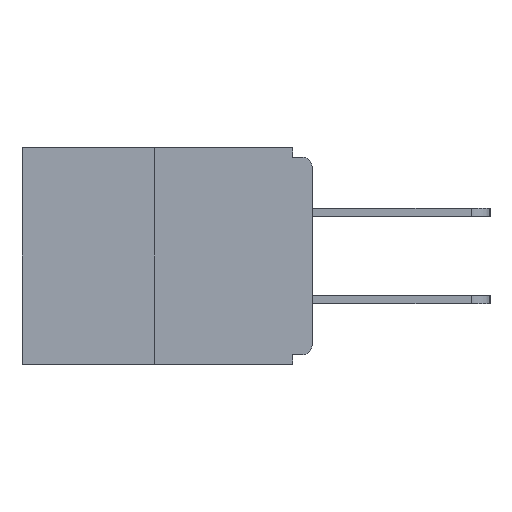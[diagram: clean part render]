
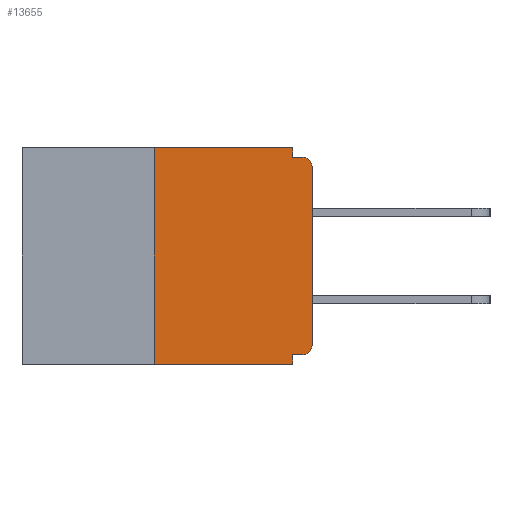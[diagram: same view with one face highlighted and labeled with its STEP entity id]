
A CAD part, left-side view. The second image highlights one B-rep face of the part: STEP entity #13655.
In plain terms, the highlighted planar face has unit normal (-1, 0, 0).
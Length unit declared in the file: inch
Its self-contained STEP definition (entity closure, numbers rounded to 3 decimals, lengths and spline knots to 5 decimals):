
#90 = VECTOR ( 'NONE', #7246, 39.37008 ) ;
#482 = CIRCLE ( 'NONE', #9554, 0.015 ) ;
#516 = DIRECTION ( 'NONE',  ( 0., 0., -1. ) ) ;
#605 = EDGE_CURVE ( 'NONE', #10616, #1938, #11566, .T. ) ;
#640 = PLANE ( 'NONE',  #7492 ) ;
#707 = EDGE_CURVE ( 'NONE', #5355, #6117, #7662, .T. ) ;
#779 = EDGE_CURVE ( 'NONE', #8005, #9842, #2909, .T. ) ;
#867 = ORIENTED_EDGE ( 'NONE', *, *, #605, .F. ) ;
#1139 = VECTOR ( 'NONE', #2866, 39.37008 ) ;
#1143 = ORIENTED_EDGE ( 'NONE', *, *, #3931, .F. ) ;
#1372 = CARTESIAN_POINT ( 'NONE',  ( 0., 0., -0.313 ) ) ;
#1499 = VECTOR ( 'NONE', #12798, 39.37008 ) ;
#1621 = CARTESIAN_POINT ( 'NONE',  ( 0., 0.031, -0.328 ) ) ;
#1938 = VERTEX_POINT ( 'NONE', #3445 ) ;
#1998 = DIRECTION ( 'NONE',  ( 0., 0., -1. ) ) ;
#2226 = CARTESIAN_POINT ( 'NONE',  ( 0., 0.46, 0. ) ) ;
#2670 = LINE ( 'NONE', #5004, #1499 ) ;
#2816 = FACE_OUTER_BOUND ( 'NONE', #9997, .T. ) ;
#2866 = DIRECTION ( 'NONE',  ( 0., 0., 1. ) ) ;
#2909 = LINE ( 'NONE', #3159, #5784 ) ;
#3020 = DIRECTION ( 'NONE',  ( 0., -1., 0. ) ) ;
#3147 = CARTESIAN_POINT ( 'NONE',  ( 0., 0.25, -0.343 ) ) ;
#3155 = VECTOR ( 'NONE', #4388, 39.37008 ) ;
#3159 = CARTESIAN_POINT ( 'NONE',  ( 0., 0., 0. ) ) ;
#3298 = ORIENTED_EDGE ( 'NONE', *, *, #13401, .T. ) ;
#3300 = EDGE_CURVE ( 'NONE', #5974, #10616, #9937, .T. ) ;
#3445 = CARTESIAN_POINT ( 'NONE',  ( 0., 0.031, -0.343 ) ) ;
#3931 = EDGE_CURVE ( 'NONE', #10969, #7299, #6026, .T. ) ;
#3944 = CARTESIAN_POINT ( 'NONE',  ( 0., 0.031, -0.015 ) ) ;
#4388 = DIRECTION ( 'NONE',  ( 0., -1., 0. ) ) ;
#4511 = VECTOR ( 'NONE', #1998, 39.37008 ) ;
#4535 = ORIENTED_EDGE ( 'NONE', *, *, #707, .F. ) ;
#4764 = DIRECTION ( 'NONE',  ( 0., 0., -1. ) ) ;
#4933 = ORIENTED_EDGE ( 'NONE', *, *, #5224, .T. ) ;
#5004 = CARTESIAN_POINT ( 'NONE',  ( 0., 0.46, -0.343 ) ) ;
#5224 = EDGE_CURVE ( 'NONE', #9842, #6117, #8707, .T. ) ;
#5355 = VERTEX_POINT ( 'NONE', #3944 ) ;
#5784 = VECTOR ( 'NONE', #12902, 39.37008 ) ;
#5789 = DIRECTION ( 'NONE',  ( 0., 1., 0. ) ) ;
#5974 = VERTEX_POINT ( 'NONE', #11361 ) ;
#6026 = LINE ( 'NONE', #7028, #1139 ) ;
#6117 = VERTEX_POINT ( 'NONE', #7425 ) ;
#6192 = CARTESIAN_POINT ( 'NONE',  ( 0., 0., -0.015 ) ) ;
#6438 = CARTESIAN_POINT ( 'NONE',  ( 0., 0.031, 0. ) ) ;
#6781 = CARTESIAN_POINT ( 'NONE',  ( 0., 0.015, -0.03 ) ) ;
#7028 = CARTESIAN_POINT ( 'NONE',  ( 0., 0.25, 0. ) ) ;
#7246 = DIRECTION ( 'NONE',  ( 0., 0., -1. ) ) ;
#7259 = CARTESIAN_POINT ( 'NONE',  ( 0., 0.46, 0. ) ) ;
#7299 = VERTEX_POINT ( 'NONE', #9845 ) ;
#7425 = CARTESIAN_POINT ( 'NONE',  ( 0., 0.015, -0.015 ) ) ;
#7492 = AXIS2_PLACEMENT_3D ( 'NONE', #7259, #9092, #516 ) ;
#7662 = LINE ( 'NONE', #6192, #9852 ) ;
#7739 = LINE ( 'NONE', #2226, #3155 ) ;
#7876 = EDGE_CURVE ( 'NONE', #7299, #9436, #7739, .T. ) ;
#8005 = VERTEX_POINT ( 'NONE', #1372 ) ;
#8116 = DIRECTION ( 'NONE',  ( 0., 0., -1. ) ) ;
#8221 = CARTESIAN_POINT ( 'NONE',  ( 0., 0.015, -0.313 ) ) ;
#8354 = DIRECTION ( 'NONE',  ( -1., 0., 0. ) ) ;
#8576 = AXIS2_PLACEMENT_3D ( 'NONE', #6781, #11177, #4764 ) ;
#8707 = CIRCLE ( 'NONE', #8576, 0.015 ) ;
#9092 = DIRECTION ( 'NONE',  ( 1., 0., 0. ) ) ;
#9436 = VERTEX_POINT ( 'NONE', #6438 ) ;
#9554 = AXIS2_PLACEMENT_3D ( 'NONE', #8221, #8354, #8116 ) ;
#9842 = VERTEX_POINT ( 'NONE', #10101 ) ;
#9845 = CARTESIAN_POINT ( 'NONE',  ( 0., 0.25, 0. ) ) ;
#9852 = VECTOR ( 'NONE', #3020, 39.37008 ) ;
#9937 = LINE ( 'NONE', #13392, #13705 ) ;
#9997 = EDGE_LOOP ( 'NONE', ( #11255, #1143, #12658, #867, #12949, #3298, #11318, #4933, #4535, #10038 ) ) ;
#10038 = ORIENTED_EDGE ( 'NONE', *, *, #13679, .F. ) ;
#10101 = CARTESIAN_POINT ( 'NONE',  ( 0., 0., -0.03 ) ) ;
#10423 = LINE ( 'NONE', #13950, #4511 ) ;
#10616 = VERTEX_POINT ( 'NONE', #1621 ) ;
#10644 = CARTESIAN_POINT ( 'NONE',  ( 0., 0.031, -0.343 ) ) ;
#10969 = VERTEX_POINT ( 'NONE', #3147 ) ;
#11177 = DIRECTION ( 'NONE',  ( -1., 0., 0. ) ) ;
#11255 = ORIENTED_EDGE ( 'NONE', *, *, #7876, .F. ) ;
#11318 = ORIENTED_EDGE ( 'NONE', *, *, #779, .T. ) ;
#11361 = CARTESIAN_POINT ( 'NONE',  ( 0., 0.015, -0.328 ) ) ;
#11566 = LINE ( 'NONE', #10644, #90 ) ;
#12658 = ORIENTED_EDGE ( 'NONE', *, *, #12970, .T. ) ;
#12798 = DIRECTION ( 'NONE',  ( 0., -1., 0. ) ) ;
#12902 = DIRECTION ( 'NONE',  ( 0., 0., 1. ) ) ;
#12949 = ORIENTED_EDGE ( 'NONE', *, *, #3300, .F. ) ;
#12970 = EDGE_CURVE ( 'NONE', #10969, #1938, #2670, .T. ) ;
#13392 = CARTESIAN_POINT ( 'NONE',  ( 0., 0., -0.328 ) ) ;
#13401 = EDGE_CURVE ( 'NONE', #5974, #8005, #482, .T. ) ;
#13655 = ADVANCED_FACE ( 'NONE', ( #2816 ), #640, .F. ) ;
#13679 = EDGE_CURVE ( 'NONE', #9436, #5355, #10423, .T. ) ;
#13705 = VECTOR ( 'NONE', #5789, 39.37008 ) ;
#13950 = CARTESIAN_POINT ( 'NONE',  ( 0., 0.031, 0. ) ) ;
